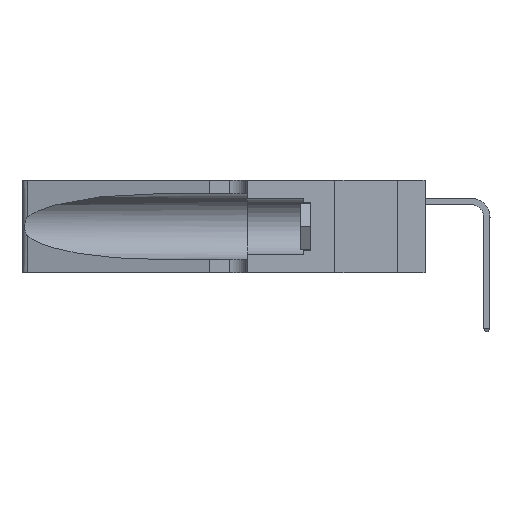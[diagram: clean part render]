
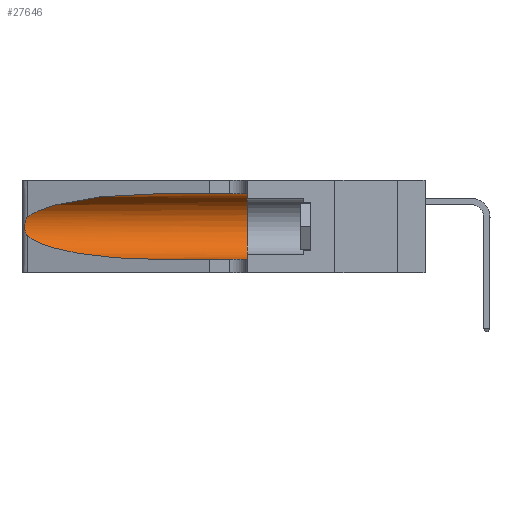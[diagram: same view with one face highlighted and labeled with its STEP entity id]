
A CAD part, left-side view. The second image highlights one B-rep face of the part: STEP entity #27646.
In plain terms, the highlighted cylindrical face has radius 3.308 mm (diameter 6.617 mm), a partial arc.
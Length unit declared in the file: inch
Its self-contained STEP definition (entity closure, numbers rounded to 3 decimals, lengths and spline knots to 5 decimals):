
#54 = CARTESIAN_POINT ( 'NONE',  ( 0.1305, 0.72297, 0.31525 ) ) ;
#318 = ORIENTED_EDGE ( 'NONE', *, *, #1251, .T. ) ;
#493 = CARTESIAN_POINT ( 'NONE',  ( 0.25487, 1.22718, 0.14631 ) ) ;
#713 = VERTEX_POINT ( 'NONE', #15376 ) ;
#1251 = EDGE_CURVE ( 'NONE', #6639, #21962, #26617, .T. ) ;
#3029 = CARTESIAN_POINT ( 'NONE',  ( 0.25487, 1.22718, 0.22369 ) ) ;
#3336 = CARTESIAN_POINT ( 'NONE',  ( 0.25639, 1.23184, 0.21858 ) ) ;
#3774 = DIRECTION ( 'NONE',  ( 0., -1., 0. ) ) ;
#3824 = CARTESIAN_POINT ( 'NONE',  ( 0.1305, 1.61858, 0.185 ) ) ;
#4803 = CYLINDRICAL_SURFACE ( 'NONE', #17304, 0.13025 ) ;
#5381 = DIRECTION ( 'NONE',  ( 0., 1., 0. ) ) ;
#5479 = CARTESIAN_POINT ( 'NONE',  ( 0.25487, 1.22718, 0.14631 ) ) ;
#6238 = CARTESIAN_POINT ( 'NONE',  ( 0.25854, 1.2359, 0.20912 ) ) ;
#6511 = EDGE_LOOP ( 'NONE', ( #318, #32955, #29639, #7917, #15119, #6726 ) ) ;
#6609 = B_SPLINE_CURVE_WITH_KNOTS ( 'NONE', 3,
 ( #23677, #17966, #3336, #23811, #6238, #26726, #9157, #29631, #12139, #32508, #15139, #35366, #18096, #493 ),
 .UNSPECIFIED., .F., .F.,
 ( 4, 2, 2, 2, 2, 2, 4 ),
 ( 0., 0.00027, 0.00053, 0.00107, 0.0016, 0.00187, 0.00214 ),
 .UNSPECIFIED. ) ;
#6626 = EDGE_CURVE ( 'NONE', #713, #15982, #32985, .T. ) ;
#6639 = VERTEX_POINT ( 'NONE', #25339 ) ;
#6726 = ORIENTED_EDGE ( 'NONE', *, *, #24054, .F. ) ;
#7917 = ORIENTED_EDGE ( 'NONE', *, *, #6626, .T. ) ;
#8130 = CARTESIAN_POINT ( 'NONE',  ( 0.1305, 0.35, 0.05475 ) ) ;
#9157 = CARTESIAN_POINT ( 'NONE',  ( 0.26075, 1.23896, 0.19203 ) ) ;
#9594 = CARTESIAN_POINT ( 'NONE',  ( 0.1305, 1.61858, 0.31525 ) ) ;
#10626 = CARTESIAN_POINT ( 'NONE',  ( 0.1305, 0.35, 0.31525 ) ) ;
#10827 = VERTEX_POINT ( 'NONE', #23377 ) ;
#11258 = CIRCLE ( 'NONE', #17369, 0.13025 ) ;
#11361 = CARTESIAN_POINT ( 'NONE',  ( 0.18966, 0.96281, 0.05475 ) ) ;
#11824 = VECTOR ( 'NONE', #3774, 39.37008 ) ;
#12139 = CARTESIAN_POINT ( 'NONE',  ( 0.26017, 1.23833, 0.17102 ) ) ;
#15119 = ORIENTED_EDGE ( 'NONE', *, *, #36720, .F. ) ;
#15139 = CARTESIAN_POINT ( 'NONE',  ( 0.25789, 1.23486, 0.15765 ) ) ;
#15142 = VERTEX_POINT ( 'NONE', #10626 ) ;
#15376 = CARTESIAN_POINT ( 'NONE',  ( 0.1305, 0.72297, 0.05475 ) ) ;
#15982 = VERTEX_POINT ( 'NONE', #8130 ) ;
#17304 = AXIS2_PLACEMENT_3D ( 'NONE', #3824, #21389, #35733 ) ;
#17369 = AXIS2_PLACEMENT_3D ( 'NONE', #22960, #5381, #25875 ) ;
#17651 = CARTESIAN_POINT ( 'NONE',  ( 0.18966, 0.96281, 0.31525 ) ) ;
#17966 = CARTESIAN_POINT ( 'NONE',  ( 0.25555, 1.22994, 0.2215 ) ) ;
#18096 = CARTESIAN_POINT ( 'NONE',  ( 0.25555, 1.22993, 0.14849 ) ) ;
#18517 = VECTOR ( 'NONE', #19487, 39.37008 ) ;
#18776 = EDGE_CURVE ( 'NONE', #21962, #10827, #6609, .T. ) ;
#19487 = DIRECTION ( 'NONE',  ( 0., -1., 0. ) ) ;
#20586 = CARTESIAN_POINT ( 'NONE',  ( 0.2373, 1.15595, 0.28018 ) ) ;
#21389 = DIRECTION ( 'NONE',  ( 0., -1., 0. ) ) ;
#21962 = VERTEX_POINT ( 'NONE', #26519 ) ;
#22960 = CARTESIAN_POINT ( 'NONE',  ( 0.1305, 0.35, 0.185 ) ) ;
#23377 = CARTESIAN_POINT ( 'NONE',  ( 0.25487, 1.22718, 0.14631 ) ) ;
#23677 = CARTESIAN_POINT ( 'NONE',  ( 0.25487, 1.22718, 0.22369 ) ) ;
#23811 = CARTESIAN_POINT ( 'NONE',  ( 0.25787, 1.23484, 0.2124 ) ) ;
#24054 = EDGE_CURVE ( 'NONE', #6639, #15142, #29201, .T. ) ;
#25107 =( BOUNDED_CURVE ( )  B_SPLINE_CURVE ( 3, ( #5479, #28879, #11361, #31756 ),
 .UNSPECIFIED., .F., .F. ) 
 B_SPLINE_CURVE_WITH_KNOTS ( ( 4, 4 ),
 ( 3.44316, 4.71239 ),
 .UNSPECIFIED. ) 
 CURVE ( )  GEOMETRIC_REPRESENTATION_ITEM ( )  RATIONAL_B_SPLINE_CURVE ( ( 1., 0.87, 0.87, 1. ) ) 
 REPRESENTATION_ITEM ( '' )  );
#25339 = CARTESIAN_POINT ( 'NONE',  ( 0.1305, 0.72297, 0.31525 ) ) ;
#25875 = DIRECTION ( 'NONE',  ( 0., 0., 1. ) ) ;
#26519 = CARTESIAN_POINT ( 'NONE',  ( 0.25487, 1.22718, 0.22369 ) ) ;
#26617 =( BOUNDED_CURVE ( )  B_SPLINE_CURVE ( 3, ( #54, #17651, #20586, #3029 ),
 .UNSPECIFIED., .F., .F. ) 
 B_SPLINE_CURVE_WITH_KNOTS ( ( 4, 4 ),
 ( 1.5708, 2.84003 ),
 .UNSPECIFIED. ) 
 CURVE ( )  GEOMETRIC_REPRESENTATION_ITEM ( )  RATIONAL_B_SPLINE_CURVE ( ( 1., 0.87, 0.87, 1. ) ) 
 REPRESENTATION_ITEM ( '' )  );
#26726 = CARTESIAN_POINT ( 'NONE',  ( 0.26018, 1.23835, 0.19895 ) ) ;
#27646 = ADVANCED_FACE ( 'NONE', ( #28151 ), #4803, .F. ) ;
#28151 = FACE_OUTER_BOUND ( 'NONE', #6511, .T. ) ;
#28879 = CARTESIAN_POINT ( 'NONE',  ( 0.2373, 1.15595, 0.08982 ) ) ;
#29201 = LINE ( 'NONE', #9594, #11824 ) ;
#29631 = CARTESIAN_POINT ( 'NONE',  ( 0.26075, 1.23896, 0.178 ) ) ;
#29639 = ORIENTED_EDGE ( 'NONE', *, *, #34348, .T. ) ;
#31756 = CARTESIAN_POINT ( 'NONE',  ( 0.1305, 0.72297, 0.05475 ) ) ;
#32508 = CARTESIAN_POINT ( 'NONE',  ( 0.25856, 1.23593, 0.16098 ) ) ;
#32955 = ORIENTED_EDGE ( 'NONE', *, *, #18776, .T. ) ;
#32985 = LINE ( 'NONE', #36750, #18517 ) ;
#34348 = EDGE_CURVE ( 'NONE', #10827, #713, #25107, .T. ) ;
#35366 = CARTESIAN_POINT ( 'NONE',  ( 0.25639, 1.23186, 0.15144 ) ) ;
#35733 = DIRECTION ( 'NONE',  ( 0., 0., -1. ) ) ;
#36720 = EDGE_CURVE ( 'NONE', #15142, #15982, #11258, .T. ) ;
#36750 = CARTESIAN_POINT ( 'NONE',  ( 0.1305, 1.61858, 0.05475 ) ) ;
